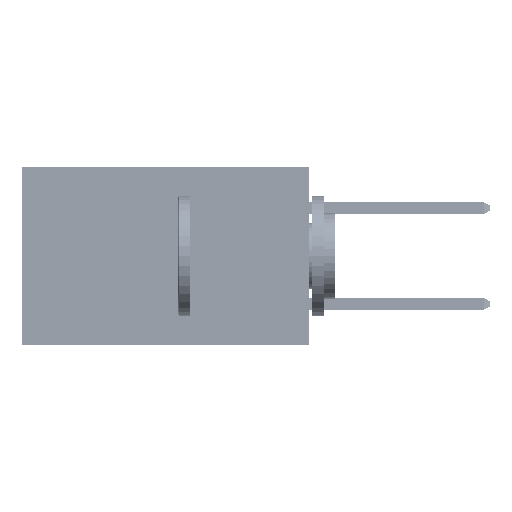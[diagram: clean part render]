
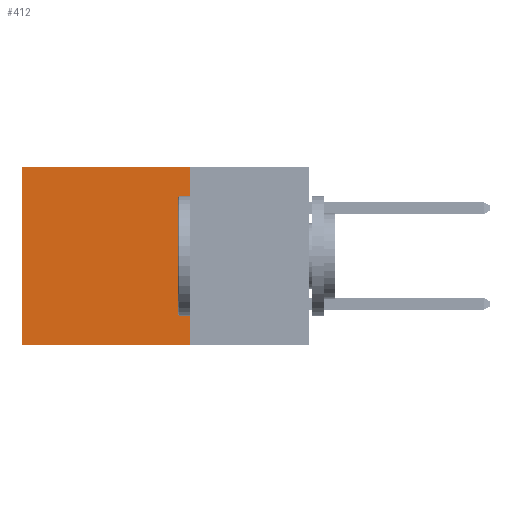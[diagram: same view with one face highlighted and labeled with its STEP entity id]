
A CAD part, left-side view. The second image highlights one B-rep face of the part: STEP entity #412.
In plain terms, the highlighted planar face has unit normal (-1, 0, 0).
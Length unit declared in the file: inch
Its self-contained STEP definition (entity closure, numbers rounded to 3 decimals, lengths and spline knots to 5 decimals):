
#412 = ADVANCED_FACE ( 'NONE', ( #37879 ), #40655, .F. ) ;
#1903 = VERTEX_POINT ( 'NONE', #47623 ) ;
#2216 = CARTESIAN_POINT ( 'NONE',  ( 0.2875, 0.25, 0. ) ) ;
#4430 = CARTESIAN_POINT ( 'NONE',  ( 0.2875, 0.6, 0. ) ) ;
#4733 = VECTOR ( 'NONE', #29928, 39.37008 ) ;
#6793 = CARTESIAN_POINT ( 'NONE',  ( 0.2875, 0.25, 0. ) ) ;
#6880 = LINE ( 'NONE', #9593, #47655 ) ;
#7356 = EDGE_LOOP ( 'NONE', ( #34368, #33177, #18739, #17323 ) ) ;
#7864 = LINE ( 'NONE', #34225, #29522 ) ;
#9593 = CARTESIAN_POINT ( 'NONE',  ( 0.2875, 0.25, 0. ) ) ;
#12228 = VERTEX_POINT ( 'NONE', #36919 ) ;
#12724 = DIRECTION ( 'NONE',  ( 1., 0., 0. ) ) ;
#13334 = LINE ( 'NONE', #4430, #44177 ) ;
#16004 = EDGE_CURVE ( 'NONE', #1903, #26898, #13334, .T. ) ;
#17323 = ORIENTED_EDGE ( 'NONE', *, *, #24403, .T. ) ;
#18739 = ORIENTED_EDGE ( 'NONE', *, *, #48072, .F. ) ;
#19098 = VERTEX_POINT ( 'NONE', #6793 ) ;
#20185 = CARTESIAN_POINT ( 'NONE',  ( 0.2875, 0.6, -0.37 ) ) ;
#20528 = DIRECTION ( 'NONE',  ( 0., 0., -1. ) ) ;
#20626 = EDGE_CURVE ( 'NONE', #12228, #26898, #7864, .T. ) ;
#21497 = DIRECTION ( 'NONE',  ( 0., 1., 0. ) ) ;
#24403 = EDGE_CURVE ( 'NONE', #19098, #1903, #6880, .T. ) ;
#26898 = VERTEX_POINT ( 'NONE', #20185 ) ;
#29522 = VECTOR ( 'NONE', #29599, 39.37008 ) ;
#29599 = DIRECTION ( 'NONE',  ( 0., 1., 0. ) ) ;
#29928 = DIRECTION ( 'NONE',  ( 0., 0., -1. ) ) ;
#33177 = ORIENTED_EDGE ( 'NONE', *, *, #20626, .F. ) ;
#34225 = CARTESIAN_POINT ( 'NONE',  ( 0.2875, 0.25, -0.37 ) ) ;
#34368 = ORIENTED_EDGE ( 'NONE', *, *, #16004, .T. ) ;
#34469 = LINE ( 'NONE', #2216, #4733 ) ;
#36342 = CARTESIAN_POINT ( 'NONE',  ( 0.2875, 0.25, 0. ) ) ;
#36919 = CARTESIAN_POINT ( 'NONE',  ( 0.2875, 0.25, -0.37 ) ) ;
#37879 = FACE_OUTER_BOUND ( 'NONE', #7356, .T. ) ;
#40141 = DIRECTION ( 'NONE',  ( 0., 0., -1. ) ) ;
#40579 = AXIS2_PLACEMENT_3D ( 'NONE', #36342, #12724, #40141 ) ;
#40655 = PLANE ( 'NONE',  #40579 ) ;
#44177 = VECTOR ( 'NONE', #20528, 39.37008 ) ;
#47623 = CARTESIAN_POINT ( 'NONE',  ( 0.2875, 0.6, 0. ) ) ;
#47655 = VECTOR ( 'NONE', #21497, 39.37008 ) ;
#48072 = EDGE_CURVE ( 'NONE', #19098, #12228, #34469, .T. ) ;
